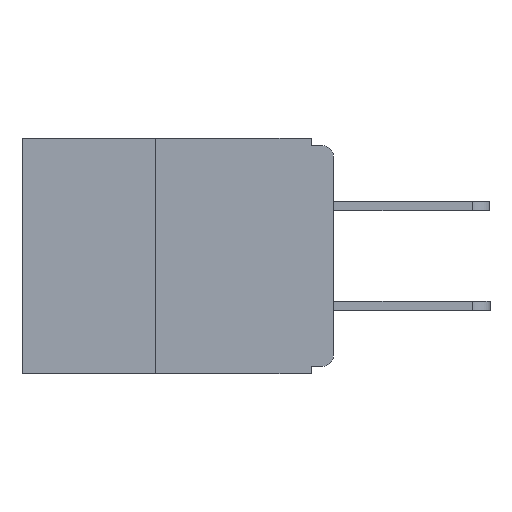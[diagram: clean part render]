
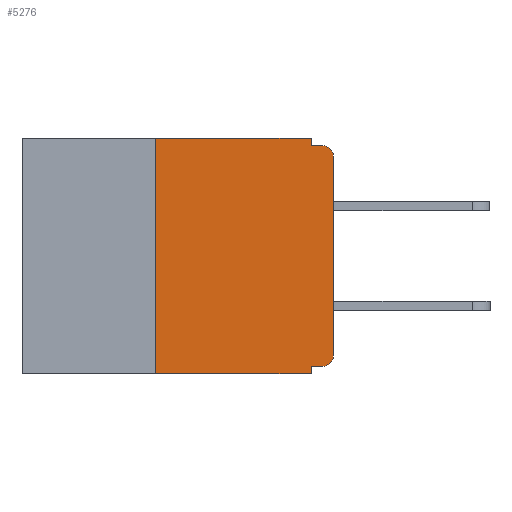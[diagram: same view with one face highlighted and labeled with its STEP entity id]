
A CAD part, left-side view. The second image highlights one B-rep face of the part: STEP entity #5276.
In plain terms, the highlighted planar face has unit normal (-1, 0, 0).
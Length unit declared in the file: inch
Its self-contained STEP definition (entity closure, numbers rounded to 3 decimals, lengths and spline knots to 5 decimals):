
#144 = VERTEX_POINT ( 'NONE', #5047 ) ;
#302 = AXIS2_PLACEMENT_3D ( 'NONE', #13938, #6427, #15189 ) ;
#379 = CARTESIAN_POINT ( 'NONE',  ( 0., 0.031, -0.32 ) ) ;
#395 = DIRECTION ( 'NONE',  ( 0., -1., 0. ) ) ;
#403 = VECTOR ( 'NONE', #3084, 39.37008 ) ;
#925 = VERTEX_POINT ( 'NONE', #5106 ) ;
#1570 = CARTESIAN_POINT ( 'NONE',  ( 0., 0.437, -0.33 ) ) ;
#1758 = VECTOR ( 'NONE', #14851, 39.37008 ) ;
#2148 = LINE ( 'NONE', #7070, #11513 ) ;
#2154 = LINE ( 'NONE', #3455, #1758 ) ;
#2343 = CARTESIAN_POINT ( 'NONE',  ( 0., 0.015, -0.01 ) ) ;
#2822 = CARTESIAN_POINT ( 'NONE',  ( 0., 0.031, 0. ) ) ;
#2992 = DIRECTION ( 'NONE',  ( 0., 0., -1. ) ) ;
#3084 = DIRECTION ( 'NONE',  ( 0., 0., 1. ) ) ;
#3141 = CARTESIAN_POINT ( 'NONE',  ( 0., 0., -0.32 ) ) ;
#3179 = CARTESIAN_POINT ( 'NONE',  ( 0., 0., -0.305 ) ) ;
#3232 = EDGE_CURVE ( 'NONE', #14991, #11579, #2148, .T. ) ;
#3395 = VECTOR ( 'NONE', #4812, 39.37008 ) ;
#3455 = CARTESIAN_POINT ( 'NONE',  ( 0., 0.031, -0.33 ) ) ;
#3563 = DIRECTION ( 'NONE',  ( 0., 0., -1. ) ) ;
#3578 = DIRECTION ( 'NONE',  ( 1., 0., 0. ) ) ;
#3600 = CARTESIAN_POINT ( 'NONE',  ( 0., 0.437, 0. ) ) ;
#3771 = PLANE ( 'NONE',  #4672 ) ;
#4454 = EDGE_CURVE ( 'NONE', #144, #11268, #11899, .T. ) ;
#4631 = ORIENTED_EDGE ( 'NONE', *, *, #3232, .F. ) ;
#4672 = AXIS2_PLACEMENT_3D ( 'NONE', #3600, #3578, #3563 ) ;
#4812 = DIRECTION ( 'NONE',  ( 0., -1., 0. ) ) ;
#4827 = ORIENTED_EDGE ( 'NONE', *, *, #11223, .F. ) ;
#4989 = ORIENTED_EDGE ( 'NONE', *, *, #10646, .T. ) ;
#5047 = CARTESIAN_POINT ( 'NONE',  ( 0., 0., -0.025 ) ) ;
#5106 = CARTESIAN_POINT ( 'NONE',  ( 0., 0.25, 0. ) ) ;
#5261 = ORIENTED_EDGE ( 'NONE', *, *, #13730, .T. ) ;
#5276 = ADVANCED_FACE ( 'NONE', ( #9334 ), #3771, .F. ) ;
#5437 = ORIENTED_EDGE ( 'NONE', *, *, #12617, .F. ) ;
#5477 = ORIENTED_EDGE ( 'NONE', *, *, #16227, .F. ) ;
#6427 = DIRECTION ( 'NONE',  ( -1., 0., 0. ) ) ;
#6431 = CIRCLE ( 'NONE', #302, 0.015 ) ;
#6544 = VECTOR ( 'NONE', #395, 39.37008 ) ;
#6809 = VERTEX_POINT ( 'NONE', #7366 ) ;
#7070 = CARTESIAN_POINT ( 'NONE',  ( 0., 0.031, 0. ) ) ;
#7117 = AXIS2_PLACEMENT_3D ( 'NONE', #14340, #14321, #14109 ) ;
#7219 = LINE ( 'NONE', #8761, #13087 ) ;
#7314 = VERTEX_POINT ( 'NONE', #3179 ) ;
#7366 = CARTESIAN_POINT ( 'NONE',  ( 0., 0.25, -0.33 ) ) ;
#7573 = ORIENTED_EDGE ( 'NONE', *, *, #4454, .T. ) ;
#7727 = ORIENTED_EDGE ( 'NONE', *, *, #15791, .F. ) ;
#8761 = CARTESIAN_POINT ( 'NONE',  ( 0., 0., 0. ) ) ;
#9334 = FACE_OUTER_BOUND ( 'NONE', #14281, .T. ) ;
#9346 = CARTESIAN_POINT ( 'NONE',  ( 0., 0., -0.01 ) ) ;
#9401 = CARTESIAN_POINT ( 'NONE',  ( 0., 0.031, -0.01 ) ) ;
#9413 = LINE ( 'NONE', #11985, #403 ) ;
#9874 = CARTESIAN_POINT ( 'NONE',  ( 0., 0.015, -0.32 ) ) ;
#9921 = LINE ( 'NONE', #9346, #6544 ) ;
#10462 = LINE ( 'NONE', #1570, #12977 ) ;
#10646 = EDGE_CURVE ( 'NONE', #7314, #144, #7219, .T. ) ;
#10738 = EDGE_CURVE ( 'NONE', #15778, #7314, #6431, .T. ) ;
#10782 = DIRECTION ( 'NONE',  ( 0., 1., 0. ) ) ;
#11223 = EDGE_CURVE ( 'NONE', #13113, #15909, #2154, .T. ) ;
#11268 = VERTEX_POINT ( 'NONE', #2343 ) ;
#11513 = VECTOR ( 'NONE', #2992, 39.37008 ) ;
#11579 = VERTEX_POINT ( 'NONE', #9401 ) ;
#11770 = DIRECTION ( 'NONE',  ( 0., -1., 0. ) ) ;
#11899 = CIRCLE ( 'NONE', #7117, 0.015 ) ;
#11985 = CARTESIAN_POINT ( 'NONE',  ( 0., 0.25, -0.33 ) ) ;
#12327 = LINE ( 'NONE', #3141, #15649 ) ;
#12380 = CARTESIAN_POINT ( 'NONE',  ( 0., 0.437, 0. ) ) ;
#12532 = DIRECTION ( 'NONE',  ( 0., 0., 1. ) ) ;
#12617 = EDGE_CURVE ( 'NONE', #11579, #11268, #9921, .T. ) ;
#12730 = LINE ( 'NONE', #12380, #3395 ) ;
#12977 = VECTOR ( 'NONE', #11770, 39.37008 ) ;
#13087 = VECTOR ( 'NONE', #12532, 39.37008 ) ;
#13113 = VERTEX_POINT ( 'NONE', #379 ) ;
#13730 = EDGE_CURVE ( 'NONE', #6809, #15909, #10462, .T. ) ;
#13938 = CARTESIAN_POINT ( 'NONE',  ( 0., 0.015, -0.305 ) ) ;
#14109 = DIRECTION ( 'NONE',  ( 0., 0., -1. ) ) ;
#14281 = EDGE_LOOP ( 'NONE', ( #4989, #7573, #5437, #4631, #7727, #5477, #5261, #4827, #14383, #14924 ) ) ;
#14321 = DIRECTION ( 'NONE',  ( -1., 0., 0. ) ) ;
#14340 = CARTESIAN_POINT ( 'NONE',  ( 0., 0.015, -0.025 ) ) ;
#14383 = ORIENTED_EDGE ( 'NONE', *, *, #16249, .F. ) ;
#14851 = DIRECTION ( 'NONE',  ( 0., 0., -1. ) ) ;
#14924 = ORIENTED_EDGE ( 'NONE', *, *, #10738, .T. ) ;
#14991 = VERTEX_POINT ( 'NONE', #2822 ) ;
#15048 = CARTESIAN_POINT ( 'NONE',  ( 0., 0.031, -0.33 ) ) ;
#15189 = DIRECTION ( 'NONE',  ( 0., 0., -1. ) ) ;
#15649 = VECTOR ( 'NONE', #10782, 39.37008 ) ;
#15778 = VERTEX_POINT ( 'NONE', #9874 ) ;
#15791 = EDGE_CURVE ( 'NONE', #925, #14991, #12730, .T. ) ;
#15909 = VERTEX_POINT ( 'NONE', #15048 ) ;
#16227 = EDGE_CURVE ( 'NONE', #6809, #925, #9413, .T. ) ;
#16249 = EDGE_CURVE ( 'NONE', #15778, #13113, #12327, .T. ) ;
